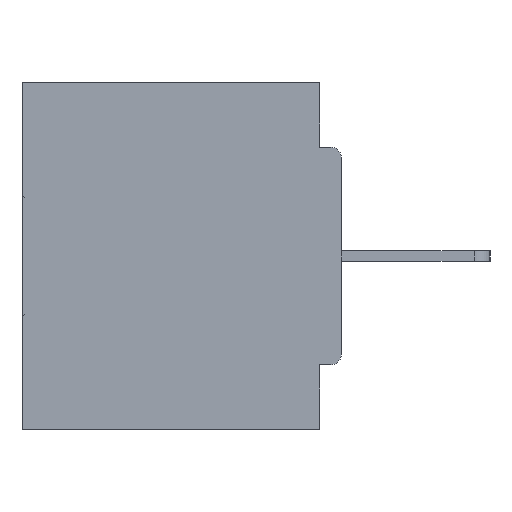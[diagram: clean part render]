
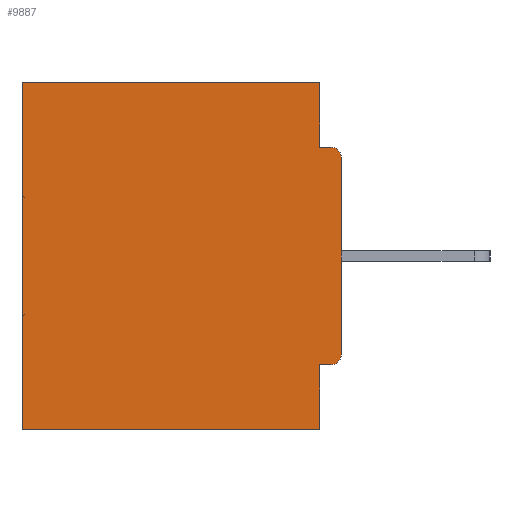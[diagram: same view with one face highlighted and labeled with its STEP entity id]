
A CAD part, left-side view. The second image highlights one B-rep face of the part: STEP entity #9887.
In plain terms, the highlighted planar face has unit normal (-1, 0, 0).
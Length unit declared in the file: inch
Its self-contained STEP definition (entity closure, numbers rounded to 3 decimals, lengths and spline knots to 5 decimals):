
#104 = ORIENTED_EDGE ( 'NONE', *, *, #36386, .F. ) ;
#943 = VERTEX_POINT ( 'NONE', #17579 ) ;
#1298 = VERTEX_POINT ( 'NONE', #32700 ) ;
#1551 = DIRECTION ( 'NONE',  ( 0., -1., 0. ) ) ;
#2039 = DIRECTION ( 'NONE',  ( -1., 0., 0. ) ) ;
#2843 = CARTESIAN_POINT ( 'NONE',  ( 0.298, 0., -0.5 ) ) ;
#2925 = EDGE_LOOP ( 'NONE', ( #27587, #6834, #23958, #33545, #26437, #11593, #19940, #104, #32181, #7257 ) ) ;
#4096 = CARTESIAN_POINT ( 'NONE',  ( 0.298, 0.031, -0.5 ) ) ;
#4222 = VECTOR ( 'NONE', #26057, 39.37008 ) ;
#4405 = CARTESIAN_POINT ( 'NONE',  ( 0.298, 0.031, -0.0935 ) ) ;
#4592 = AXIS2_PLACEMENT_3D ( 'NONE', #19397, #2039, #22292 ) ;
#4810 = LINE ( 'NONE', #26304, #19302 ) ;
#6089 = VERTEX_POINT ( 'NONE', #31015 ) ;
#6834 = ORIENTED_EDGE ( 'NONE', *, *, #26482, .F. ) ;
#7257 = ORIENTED_EDGE ( 'NONE', *, *, #21577, .F. ) ;
#7802 = DIRECTION ( 'NONE',  ( -1., 0., 0. ) ) ;
#8946 = EDGE_CURVE ( 'NONE', #6089, #1298, #13059, .T. ) ;
#9147 = CARTESIAN_POINT ( 'NONE',  ( 0.298, 0.031, -0.5 ) ) ;
#9887 = ADVANCED_FACE ( 'NONE', ( #19721 ), #26610, .F. ) ;
#11593 = ORIENTED_EDGE ( 'NONE', *, *, #27888, .F. ) ;
#13059 = LINE ( 'NONE', #33716, #27418 ) ;
#13083 = VERTEX_POINT ( 'NONE', #25096 ) ;
#13343 = VERTEX_POINT ( 'NONE', #14796 ) ;
#14796 = CARTESIAN_POINT ( 'NONE',  ( 0.298, 0.031, -0.4065 ) ) ;
#15084 = LINE ( 'NONE', #18991, #30297 ) ;
#15214 = DIRECTION ( 'NONE',  ( 1., 0., 0. ) ) ;
#15861 = LINE ( 'NONE', #2843, #23518 ) ;
#16411 = VERTEX_POINT ( 'NONE', #4405 ) ;
#16905 = EDGE_CURVE ( 'NONE', #28034, #16411, #18582, .T. ) ;
#16984 = VERTEX_POINT ( 'NONE', #29998 ) ;
#17579 = CARTESIAN_POINT ( 'NONE',  ( 0.298, 0., -0.1085 ) ) ;
#17943 = VECTOR ( 'NONE', #27175, 39.37008 ) ;
#18170 = AXIS2_PLACEMENT_3D ( 'NONE', #32189, #15214, #35157 ) ;
#18582 = LINE ( 'NONE', #4096, #17943 ) ;
#18991 = CARTESIAN_POINT ( 'NONE',  ( 0.298, 0., 0. ) ) ;
#19302 = VECTOR ( 'NONE', #23579, 39.37008 ) ;
#19397 = CARTESIAN_POINT ( 'NONE',  ( 0.298, 0.015, -0.3915 ) ) ;
#19466 = EDGE_CURVE ( 'NONE', #13083, #16984, #34909, .T. ) ;
#19721 = FACE_OUTER_BOUND ( 'NONE', #2925, .T. ) ;
#19940 = ORIENTED_EDGE ( 'NONE', *, *, #23408, .F. ) ;
#21577 = EDGE_CURVE ( 'NONE', #943, #16984, #31244, .T. ) ;
#22292 = DIRECTION ( 'NONE',  ( 0., 0., -1. ) ) ;
#22858 = CIRCLE ( 'NONE', #32756, 0.015 ) ;
#23099 = DIRECTION ( 'NONE',  ( 0., 1., 0. ) ) ;
#23191 = CARTESIAN_POINT ( 'NONE',  ( 0.298, 0., -0.4065 ) ) ;
#23408 = EDGE_CURVE ( 'NONE', #13343, #34027, #4810, .T. ) ;
#23518 = VECTOR ( 'NONE', #23099, 39.37008 ) ;
#23579 = DIRECTION ( 'NONE',  ( 0., 0., -1. ) ) ;
#23592 = DIRECTION ( 'NONE',  ( 0., 0., -1. ) ) ;
#23723 = VECTOR ( 'NONE', #23592, 39.37008 ) ;
#23958 = ORIENTED_EDGE ( 'NONE', *, *, #16905, .F. ) ;
#24344 = CARTESIAN_POINT ( 'NONE',  ( 0.298, 0.015, -0.0935 ) ) ;
#25049 = CARTESIAN_POINT ( 'NONE',  ( 0.298, 0.015, -0.1085 ) ) ;
#25096 = CARTESIAN_POINT ( 'NONE',  ( 0.298, 0.015, -0.4065 ) ) ;
#25312 = DIRECTION ( 'NONE',  ( 0., 0., -1. ) ) ;
#25783 = LINE ( 'NONE', #30411, #32433 ) ;
#26057 = DIRECTION ( 'NONE',  ( 0., 1., 0. ) ) ;
#26304 = CARTESIAN_POINT ( 'NONE',  ( 0.298, 0.031, -0.5 ) ) ;
#26437 = ORIENTED_EDGE ( 'NONE', *, *, #8946, .T. ) ;
#26482 = EDGE_CURVE ( 'NONE', #16411, #28146, #25783, .T. ) ;
#26610 = PLANE ( 'NONE',  #18170 ) ;
#27175 = DIRECTION ( 'NONE',  ( 0., 0., -1. ) ) ;
#27249 = LINE ( 'NONE', #23191, #4222 ) ;
#27418 = VECTOR ( 'NONE', #25312, 39.37008 ) ;
#27587 = ORIENTED_EDGE ( 'NONE', *, *, #34858, .T. ) ;
#27654 = DIRECTION ( 'NONE',  ( 0., 1., 0. ) ) ;
#27888 = EDGE_CURVE ( 'NONE', #34027, #1298, #15861, .T. ) ;
#27916 = DIRECTION ( 'NONE',  ( 0., 0., -1. ) ) ;
#28034 = VERTEX_POINT ( 'NONE', #32265 ) ;
#28146 = VERTEX_POINT ( 'NONE', #24344 ) ;
#29998 = CARTESIAN_POINT ( 'NONE',  ( 0.298, 0., -0.3915 ) ) ;
#30297 = VECTOR ( 'NONE', #27654, 39.37008 ) ;
#30411 = CARTESIAN_POINT ( 'NONE',  ( 0.298, 0., -0.0935 ) ) ;
#31015 = CARTESIAN_POINT ( 'NONE',  ( 0.298, 0.46, 0. ) ) ;
#31244 = LINE ( 'NONE', #34755, #23723 ) ;
#32181 = ORIENTED_EDGE ( 'NONE', *, *, #19466, .T. ) ;
#32189 = CARTESIAN_POINT ( 'NONE',  ( 0.298, 0., 0. ) ) ;
#32265 = CARTESIAN_POINT ( 'NONE',  ( 0.298, 0.031, 0. ) ) ;
#32433 = VECTOR ( 'NONE', #1551, 39.37008 ) ;
#32700 = CARTESIAN_POINT ( 'NONE',  ( 0.298, 0.46, -0.5 ) ) ;
#32756 = AXIS2_PLACEMENT_3D ( 'NONE', #25049, #7802, #27916 ) ;
#33545 = ORIENTED_EDGE ( 'NONE', *, *, #36895, .T. ) ;
#33716 = CARTESIAN_POINT ( 'NONE',  ( 0.298, 0.46, 0. ) ) ;
#34027 = VERTEX_POINT ( 'NONE', #9147 ) ;
#34755 = CARTESIAN_POINT ( 'NONE',  ( 0.298, 0., 0. ) ) ;
#34858 = EDGE_CURVE ( 'NONE', #943, #28146, #22858, .T. ) ;
#34909 = CIRCLE ( 'NONE', #4592, 0.015 ) ;
#35157 = DIRECTION ( 'NONE',  ( 0., 0., -1. ) ) ;
#36386 = EDGE_CURVE ( 'NONE', #13083, #13343, #27249, .T. ) ;
#36895 = EDGE_CURVE ( 'NONE', #28034, #6089, #15084, .T. ) ;
